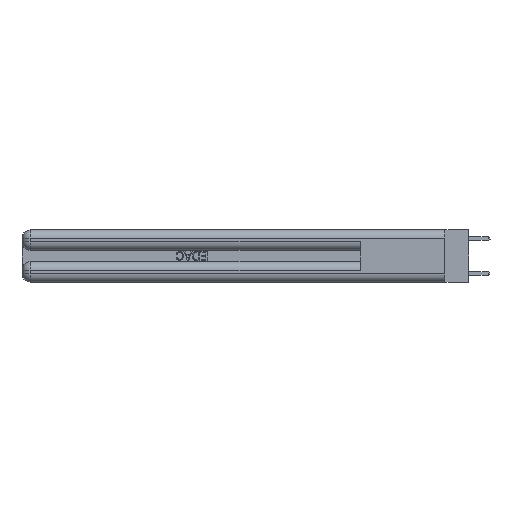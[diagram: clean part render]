
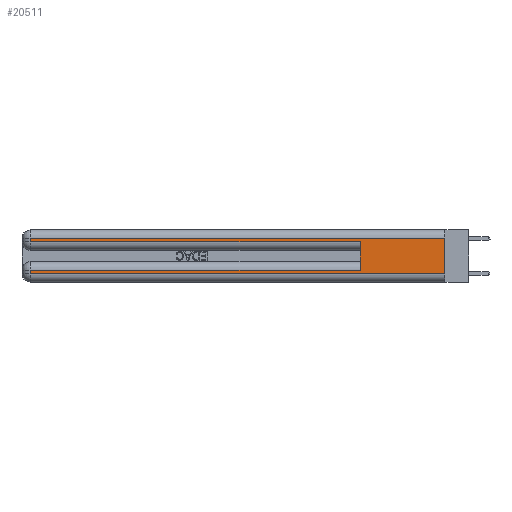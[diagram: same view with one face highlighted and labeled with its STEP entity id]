
A CAD part, left-side view. The second image highlights one B-rep face of the part: STEP entity #20511.
In plain terms, the highlighted planar face has unit normal (-1, 0, 0).
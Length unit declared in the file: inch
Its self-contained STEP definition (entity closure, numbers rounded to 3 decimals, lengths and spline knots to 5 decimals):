
#835 = VECTOR ( 'NONE', #10866, 39.37008 ) ;
#1371 = DIRECTION ( 'NONE',  ( 0., 1., 0. ) ) ;
#2090 = EDGE_LOOP ( 'NONE', ( #25986, #27055, #12979, #24976, #17381, #9627, #26324, #3979 ) ) ;
#3003 = LINE ( 'NONE', #8589, #8853 ) ;
#3357 = VECTOR ( 'NONE', #15768, 39.37008 ) ;
#3979 = ORIENTED_EDGE ( 'NONE', *, *, #26400, .T. ) ;
#4296 = PLANE ( 'NONE',  #18248 ) ;
#4332 = VECTOR ( 'NONE', #31725, 39.37008 ) ;
#5906 = LINE ( 'NONE', #22023, #4332 ) ;
#6262 = LINE ( 'NONE', #14986, #30617 ) ;
#7040 = CARTESIAN_POINT ( 'NONE',  ( 0., 2.94, 0.085 ) ) ;
#8368 = CARTESIAN_POINT ( 'NONE',  ( 0., 2.94, 0.37 ) ) ;
#8447 = CARTESIAN_POINT ( 'NONE',  ( 0., 0.6, 0.085 ) ) ;
#8589 = CARTESIAN_POINT ( 'NONE',  ( 0., 0., 0.37 ) ) ;
#8641 = EDGE_CURVE ( 'NONE', #26651, #17771, #9652, .T. ) ;
#8853 = VECTOR ( 'NONE', #28048, 39.37008 ) ;
#9211 = EDGE_CURVE ( 'NONE', #19046, #22653, #19545, .T. ) ;
#9627 = ORIENTED_EDGE ( 'NONE', *, *, #8641, .T. ) ;
#9652 = LINE ( 'NONE', #26359, #16197 ) ;
#10417 = VERTEX_POINT ( 'NONE', #13478 ) ;
#10866 = DIRECTION ( 'NONE',  ( 0., 0., -1. ) ) ;
#11765 = DIRECTION ( 'NONE',  ( 1., 0., 0. ) ) ;
#11839 = DIRECTION ( 'NONE',  ( 0., 1., 0. ) ) ;
#12478 = CARTESIAN_POINT ( 'NONE',  ( 0., 0., 0.31 ) ) ;
#12979 = ORIENTED_EDGE ( 'NONE', *, *, #13643, .T. ) ;
#13122 = VECTOR ( 'NONE', #1371, 39.37008 ) ;
#13478 = CARTESIAN_POINT ( 'NONE',  ( 0., 2.94, 0.06 ) ) ;
#13643 = EDGE_CURVE ( 'NONE', #22653, #31709, #20513, .T. ) ;
#13994 = CARTESIAN_POINT ( 'NONE',  ( 0., 2.94, 0.31 ) ) ;
#14697 = CARTESIAN_POINT ( 'NONE',  ( 0., 2.94, 0.285 ) ) ;
#14986 = CARTESIAN_POINT ( 'NONE',  ( 0., 0.6, 0.145 ) ) ;
#15768 = DIRECTION ( 'NONE',  ( 0., 0., -1. ) ) ;
#16197 = VECTOR ( 'NONE', #11839, 39.37008 ) ;
#16458 = LINE ( 'NONE', #24805, #28569 ) ;
#17245 = LINE ( 'NONE', #27810, #3357 ) ;
#17381 = ORIENTED_EDGE ( 'NONE', *, *, #27054, .F. ) ;
#17413 = DIRECTION ( 'NONE',  ( 0., 0., 1. ) ) ;
#17614 = CARTESIAN_POINT ( 'NONE',  ( 0., 0.6, 0.285 ) ) ;
#17771 = VERTEX_POINT ( 'NONE', #7040 ) ;
#18248 = AXIS2_PLACEMENT_3D ( 'NONE', #26278, #11765, #28735 ) ;
#19046 = VERTEX_POINT ( 'NONE', #12478 ) ;
#19545 = LINE ( 'NONE', #30665, #13122 ) ;
#20235 = VERTEX_POINT ( 'NONE', #22598 ) ;
#20511 = ADVANCED_FACE ( 'NONE', ( #30915 ), #4296, .F. ) ;
#20513 = LINE ( 'NONE', #8368, #835 ) ;
#21526 = EDGE_CURVE ( 'NONE', #17771, #10417, #17245, .T. ) ;
#21984 = EDGE_CURVE ( 'NONE', #31709, #27117, #16458, .T. ) ;
#22023 = CARTESIAN_POINT ( 'NONE',  ( 0., 0., 0.06 ) ) ;
#22598 = CARTESIAN_POINT ( 'NONE',  ( 0., 0., 0.06 ) ) ;
#22653 = VERTEX_POINT ( 'NONE', #13994 ) ;
#24805 = CARTESIAN_POINT ( 'NONE',  ( 0., 0., 0.285 ) ) ;
#24976 = ORIENTED_EDGE ( 'NONE', *, *, #21984, .T. ) ;
#25986 = ORIENTED_EDGE ( 'NONE', *, *, #31357, .F. ) ;
#26278 = CARTESIAN_POINT ( 'NONE',  ( 0., 0., 0.37 ) ) ;
#26324 = ORIENTED_EDGE ( 'NONE', *, *, #21526, .T. ) ;
#26359 = CARTESIAN_POINT ( 'NONE',  ( 0., 0., 0.085 ) ) ;
#26400 = EDGE_CURVE ( 'NONE', #10417, #20235, #5906, .T. ) ;
#26651 = VERTEX_POINT ( 'NONE', #8447 ) ;
#27054 = EDGE_CURVE ( 'NONE', #26651, #27117, #6262, .T. ) ;
#27055 = ORIENTED_EDGE ( 'NONE', *, *, #9211, .T. ) ;
#27117 = VERTEX_POINT ( 'NONE', #17614 ) ;
#27249 = DIRECTION ( 'NONE',  ( 0., -1., 0. ) ) ;
#27810 = CARTESIAN_POINT ( 'NONE',  ( 0., 2.94, 0.37 ) ) ;
#28048 = DIRECTION ( 'NONE',  ( 0., 0., -1. ) ) ;
#28569 = VECTOR ( 'NONE', #27249, 39.37008 ) ;
#28735 = DIRECTION ( 'NONE',  ( 0., 0., -1. ) ) ;
#30617 = VECTOR ( 'NONE', #17413, 39.37008 ) ;
#30665 = CARTESIAN_POINT ( 'NONE',  ( 0., 0., 0.31 ) ) ;
#30915 = FACE_OUTER_BOUND ( 'NONE', #2090, .T. ) ;
#31357 = EDGE_CURVE ( 'NONE', #19046, #20235, #3003, .T. ) ;
#31709 = VERTEX_POINT ( 'NONE', #14697 ) ;
#31725 = DIRECTION ( 'NONE',  ( 0., -1., 0. ) ) ;
